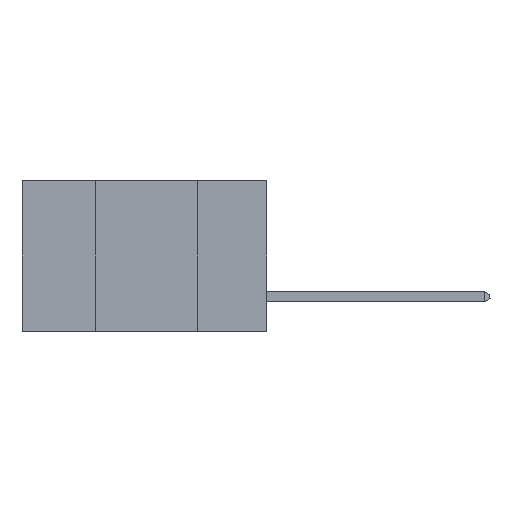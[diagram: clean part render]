
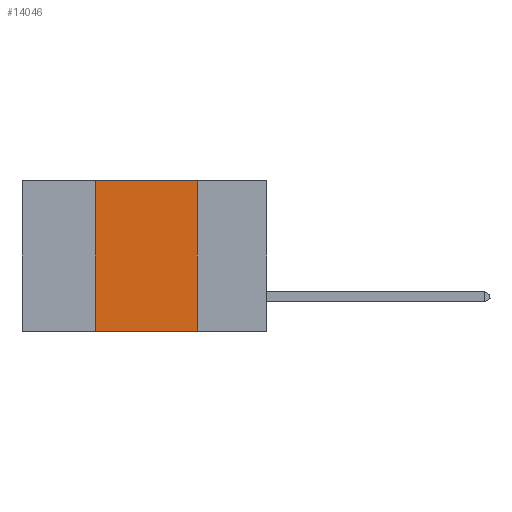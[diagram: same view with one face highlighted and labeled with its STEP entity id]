
A CAD part, left-side view. The second image highlights one B-rep face of the part: STEP entity #14046.
In plain terms, the highlighted planar face has unit normal (-1, 0, 0).
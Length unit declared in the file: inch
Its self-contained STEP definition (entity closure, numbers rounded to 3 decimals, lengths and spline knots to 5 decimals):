
#1059 = EDGE_CURVE ( 'NONE', #6255, #7104, #3231, .T. ) ;
#1449 = PLANE ( 'NONE',  #3917 ) ;
#1622 = CARTESIAN_POINT ( 'NONE',  ( 0., 0.17, 0. ) ) ;
#2183 = VECTOR ( 'NONE', #10347, 39.37008 ) ;
#2573 = CARTESIAN_POINT ( 'NONE',  ( 0., 0.17, -0.37 ) ) ;
#2808 = CARTESIAN_POINT ( 'NONE',  ( 0., 0.42, 0. ) ) ;
#2866 = CARTESIAN_POINT ( 'NONE',  ( 0., 0.42, -0.37 ) ) ;
#3231 = LINE ( 'NONE', #14351, #6929 ) ;
#3479 = ORIENTED_EDGE ( 'NONE', *, *, #4868, .F. ) ;
#3717 = ORIENTED_EDGE ( 'NONE', *, *, #1059, .T. ) ;
#3917 = AXIS2_PLACEMENT_3D ( 'NONE', #4921, #17653, #15987 ) ;
#4348 = DIRECTION ( 'NONE',  ( 0., 0., 1. ) ) ;
#4868 = EDGE_CURVE ( 'NONE', #6255, #6082, #13213, .T. ) ;
#4921 = CARTESIAN_POINT ( 'NONE',  ( 0., 0.6, 0. ) ) ;
#5614 = ORIENTED_EDGE ( 'NONE', *, *, #11438, .F. ) ;
#6082 = VERTEX_POINT ( 'NONE', #7676 ) ;
#6255 = VERTEX_POINT ( 'NONE', #2866 ) ;
#6425 = EDGE_CURVE ( 'NONE', #6082, #14197, #11321, .T. ) ;
#6929 = VECTOR ( 'NONE', #15889, 39.37008 ) ;
#7104 = VERTEX_POINT ( 'NONE', #2573 ) ;
#7604 = VECTOR ( 'NONE', #14547, 39.37008 ) ;
#7676 = CARTESIAN_POINT ( 'NONE',  ( 0., 0.42, 0. ) ) ;
#8444 = VECTOR ( 'NONE', #4348, 39.37008 ) ;
#10347 = DIRECTION ( 'NONE',  ( 0., -1., 0. ) ) ;
#11321 = LINE ( 'NONE', #18355, #2183 ) ;
#11438 = EDGE_CURVE ( 'NONE', #14197, #7104, #19577, .T. ) ;
#12502 = FACE_OUTER_BOUND ( 'NONE', #18639, .T. ) ;
#13213 = LINE ( 'NONE', #2808, #8444 ) ;
#13709 = ORIENTED_EDGE ( 'NONE', *, *, #6425, .F. ) ;
#14046 = ADVANCED_FACE ( 'NONE', ( #12502 ), #1449, .F. ) ;
#14197 = VERTEX_POINT ( 'NONE', #15395 ) ;
#14351 = CARTESIAN_POINT ( 'NONE',  ( 0., 0.6, -0.37 ) ) ;
#14547 = DIRECTION ( 'NONE',  ( 0., 0., -1. ) ) ;
#15395 = CARTESIAN_POINT ( 'NONE',  ( 0., 0.17, 0. ) ) ;
#15889 = DIRECTION ( 'NONE',  ( 0., -1., 0. ) ) ;
#15987 = DIRECTION ( 'NONE',  ( 0., 0., -1. ) ) ;
#17653 = DIRECTION ( 'NONE',  ( 1., 0., 0. ) ) ;
#18355 = CARTESIAN_POINT ( 'NONE',  ( 0., 0.6, 0. ) ) ;
#18639 = EDGE_LOOP ( 'NONE', ( #5614, #13709, #3479, #3717 ) ) ;
#19577 = LINE ( 'NONE', #1622, #7604 ) ;
